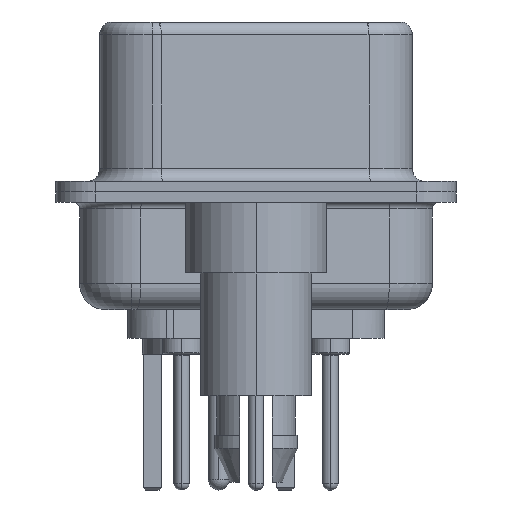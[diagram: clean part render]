
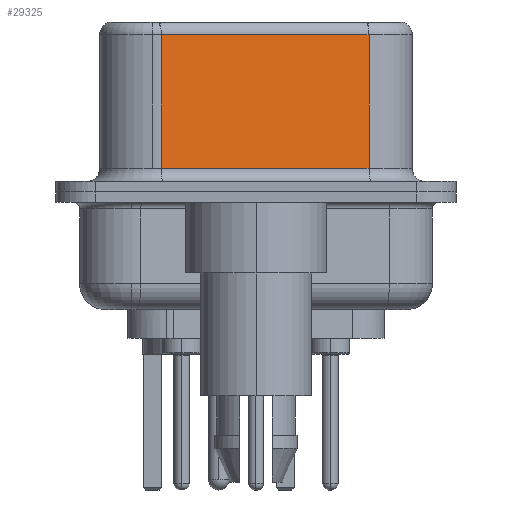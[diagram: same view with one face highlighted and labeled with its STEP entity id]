
A CAD part, left-side view. The second image highlights one B-rep face of the part: STEP entity #29325.
In plain terms, the highlighted planar face has unit normal (-0.985, -0.174, 0).
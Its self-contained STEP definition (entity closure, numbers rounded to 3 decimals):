
#2024 = CARTESIAN_POINT ( 'NONE',  ( 5.132, -4.322, 0.9 ) ) ;
#2050 = LINE ( 'NONE', #21719, #13264 ) ;
#2659 = CARTESIAN_POINT ( 'NONE',  ( 3.73, 3.628, 0.9 ) ) ;
#3476 = VERTEX_POINT ( 'NONE', #2659 ) ;
#4597 = DIRECTION ( 'NONE',  ( 0.174, -0.985, 0. ) ) ;
#4875 = CARTESIAN_POINT ( 'NONE',  ( 5.132, -4.322, 0.9 ) ) ;
#4949 = CARTESIAN_POINT ( 'NONE',  ( 5.132, -4.322, 6.52 ) ) ;
#5205 = DIRECTION ( 'NONE',  ( 0.985, 0.174, 0. ) ) ;
#6047 = FACE_OUTER_BOUND ( 'NONE', #10357, .T. ) ;
#7393 = LINE ( 'NONE', #4949, #26872 ) ;
#7532 = VERTEX_POINT ( 'NONE', #4875 ) ;
#7817 = CARTESIAN_POINT ( 'NONE',  ( 5.132, -4.322, 6.52 ) ) ;
#9036 = VERTEX_POINT ( 'NONE', #18816 ) ;
#9708 = EDGE_CURVE ( 'NONE', #9036, #3476, #2050, .T. ) ;
#10357 = EDGE_LOOP ( 'NONE', ( #10813, #26870, #26732, #16517 ) ) ;
#10813 = ORIENTED_EDGE ( 'NONE', *, *, #27347, .F. ) ;
#13264 = VECTOR ( 'NONE', #21691, 1000. ) ;
#16189 = LINE ( 'NONE', #2024, #22151 ) ;
#16517 = ORIENTED_EDGE ( 'NONE', *, *, #20599, .T. ) ;
#18816 = CARTESIAN_POINT ( 'NONE',  ( 3.73, 3.628, 6.02 ) ) ;
#19094 = CARTESIAN_POINT ( 'NONE',  ( 5.132, -4.322, 6.02 ) ) ;
#20599 = EDGE_CURVE ( 'NONE', #3476, #7532, #16189, .T. ) ;
#21139 = CARTESIAN_POINT ( 'NONE',  ( 5.132, -4.322, 6.02 ) ) ;
#21691 = DIRECTION ( 'NONE',  ( 0., 0., -1. ) ) ;
#21693 = DIRECTION ( 'NONE',  ( -0.174, 0.985, 0. ) ) ;
#21719 = CARTESIAN_POINT ( 'NONE',  ( 3.73, 3.628, 6.52 ) ) ;
#22151 = VECTOR ( 'NONE', #4597, 1000. ) ;
#25811 = VECTOR ( 'NONE', #21693, 1000. ) ;
#26598 = LINE ( 'NONE', #19094, #25811 ) ;
#26732 = ORIENTED_EDGE ( 'NONE', *, *, #9708, .T. ) ;
#26870 = ORIENTED_EDGE ( 'NONE', *, *, #32824, .T. ) ;
#26872 = VECTOR ( 'NONE', #30436, 1000. ) ;
#27347 = EDGE_CURVE ( 'NONE', #32670, #7532, #7393, .T. ) ;
#28134 = PLANE ( 'NONE',  #31673 ) ;
#29325 = ADVANCED_FACE ( 'NONE', ( #6047 ), #28134, .F. ) ;
#30436 = DIRECTION ( 'NONE',  ( 0., 0., -1. ) ) ;
#30724 = DIRECTION ( 'NONE',  ( -0.174, 0.985, 0. ) ) ;
#31673 = AXIS2_PLACEMENT_3D ( 'NONE', #7817, #5205, #30724 ) ;
#32670 = VERTEX_POINT ( 'NONE', #21139 ) ;
#32824 = EDGE_CURVE ( 'NONE', #32670, #9036, #26598, .T. ) ;
